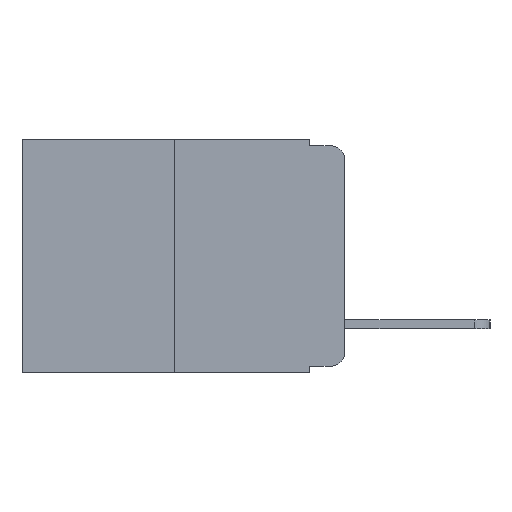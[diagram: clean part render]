
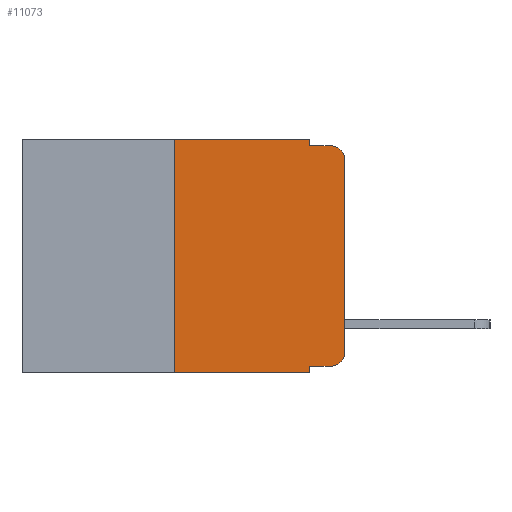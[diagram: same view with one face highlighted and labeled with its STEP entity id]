
A CAD part, left-side view. The second image highlights one B-rep face of the part: STEP entity #11073.
In plain terms, the highlighted planar face has unit normal (-1, 0, 0).
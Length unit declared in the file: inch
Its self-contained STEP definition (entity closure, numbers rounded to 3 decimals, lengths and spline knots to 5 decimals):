
#150 = CARTESIAN_POINT ( 'NONE',  ( 0., 0.051, -0.333 ) ) ;
#694 = CARTESIAN_POINT ( 'NONE',  ( 0., 0.051, -0.343 ) ) ;
#814 = DIRECTION ( 'NONE',  ( 0., -1., 0. ) ) ;
#2095 = DIRECTION ( 'NONE',  ( 0., -1., 0. ) ) ;
#2851 = LINE ( 'NONE', #6219, #6591 ) ;
#3187 = VERTEX_POINT ( 'NONE', #4512 ) ;
#4358 = EDGE_CURVE ( 'NONE', #10413, #14673, #15029, .T. ) ;
#4512 = CARTESIAN_POINT ( 'NONE',  ( 0., 0.051, -0.333 ) ) ;
#5055 = DIRECTION ( 'NONE',  ( 0., -1., 0. ) ) ;
#5499 = VERTEX_POINT ( 'NONE', #18610 ) ;
#5692 = LINE ( 'NONE', #6854, #15214 ) ;
#6219 = CARTESIAN_POINT ( 'NONE',  ( 0., 0.473, 0. ) ) ;
#6591 = VECTOR ( 'NONE', #15666, 39.37008 ) ;
#6714 = CARTESIAN_POINT ( 'NONE',  ( 0., 0., -0.03 ) ) ;
#6854 = CARTESIAN_POINT ( 'NONE',  ( 0., 0.473, -0.343 ) ) ;
#7719 = CARTESIAN_POINT ( 'NONE',  ( 0., 0.02, -0.03 ) ) ;
#7760 = ORIENTED_EDGE ( 'NONE', *, *, #13762, .T. ) ;
#7938 = ORIENTED_EDGE ( 'NONE', *, *, #14966, .T. ) ;
#8067 = ORIENTED_EDGE ( 'NONE', *, *, #16184, .F. ) ;
#8195 = ORIENTED_EDGE ( 'NONE', *, *, #19721, .F. ) ;
#8263 = DIRECTION ( 'NONE',  ( 0., 0., -1. ) ) ;
#8351 = ORIENTED_EDGE ( 'NONE', *, *, #21509, .F. ) ;
#8420 = VECTOR ( 'NONE', #19417, 39.37008 ) ;
#8517 = CARTESIAN_POINT ( 'NONE',  ( 0., 0.25, 0. ) ) ;
#8689 = LINE ( 'NONE', #17704, #18044 ) ;
#8781 = ORIENTED_EDGE ( 'NONE', *, *, #4358, .F. ) ;
#8802 = ORIENTED_EDGE ( 'NONE', *, *, #21720, .T. ) ;
#8980 = ORIENTED_EDGE ( 'NONE', *, *, #10697, .F. ) ;
#9403 = ORIENTED_EDGE ( 'NONE', *, *, #10216, .T. ) ;
#9608 = ORIENTED_EDGE ( 'NONE', *, *, #9860, .T. ) ;
#9687 = DIRECTION ( 'NONE',  ( 0., 0., -1. ) ) ;
#9860 = EDGE_CURVE ( 'NONE', #12364, #5499, #10754, .T. ) ;
#9892 = CARTESIAN_POINT ( 'NONE',  ( 0., 0.473, 0. ) ) ;
#10216 = EDGE_CURVE ( 'NONE', #3187, #12364, #19319, .T. ) ;
#10413 = VERTEX_POINT ( 'NONE', #12498 ) ;
#10498 = DIRECTION ( 'NONE',  ( 0., 0., 1. ) ) ;
#10518 = EDGE_LOOP ( 'NONE', ( #7760, #7938, #8067, #8195, #8351, #8781, #8802, #8980, #9403, #9608 ) ) ;
#10697 = EDGE_CURVE ( 'NONE', #3187, #17299, #8689, .T. ) ;
#10754 = CIRCLE ( 'NONE', #13835, 0.02 ) ;
#10838 = CARTESIAN_POINT ( 'NONE',  ( 0., 0., 0. ) ) ;
#11073 = ADVANCED_FACE ( 'NONE', ( #19143 ), #20799, .F. ) ;
#11383 = DIRECTION ( 'NONE',  ( -1., 0., 0. ) ) ;
#11640 = AXIS2_PLACEMENT_3D ( 'NONE', #9892, #22501, #11846 ) ;
#11846 = DIRECTION ( 'NONE',  ( 0., 0., -1. ) ) ;
#12173 = DIRECTION ( 'NONE',  ( 0., 0., -1. ) ) ;
#12201 = CARTESIAN_POINT ( 'NONE',  ( 0., 0.051, -0.01 ) ) ;
#12364 = VERTEX_POINT ( 'NONE', #14083 ) ;
#12498 = CARTESIAN_POINT ( 'NONE',  ( 0., 0.25, -0.343 ) ) ;
#12636 = CARTESIAN_POINT ( 'NONE',  ( 0., 0.25, 0. ) ) ;
#13213 = VERTEX_POINT ( 'NONE', #14262 ) ;
#13762 = EDGE_CURVE ( 'NONE', #5499, #20594, #17662, .T. ) ;
#13835 = AXIS2_PLACEMENT_3D ( 'NONE', #22118, #11383, #12173 ) ;
#14083 = CARTESIAN_POINT ( 'NONE',  ( 0., 0.02, -0.333 ) ) ;
#14163 = LINE ( 'NONE', #21128, #8420 ) ;
#14262 = CARTESIAN_POINT ( 'NONE',  ( 0., 0.051, 0. ) ) ;
#14574 = VECTOR ( 'NONE', #2095, 39.37008 ) ;
#14673 = VERTEX_POINT ( 'NONE', #12636 ) ;
#14966 = EDGE_CURVE ( 'NONE', #20594, #16890, #17603, .T. ) ;
#15012 = VERTEX_POINT ( 'NONE', #17270 ) ;
#15029 = LINE ( 'NONE', #8517, #23692 ) ;
#15214 = VECTOR ( 'NONE', #5055, 39.37008 ) ;
#15666 = DIRECTION ( 'NONE',  ( 0., -1., 0. ) ) ;
#15860 = VECTOR ( 'NONE', #814, 39.37008 ) ;
#16184 = EDGE_CURVE ( 'NONE', #15012, #16890, #19993, .T. ) ;
#16391 = DIRECTION ( 'NONE',  ( 0., 0., 1. ) ) ;
#16580 = AXIS2_PLACEMENT_3D ( 'NONE', #7719, #20627, #9687 ) ;
#16890 = VERTEX_POINT ( 'NONE', #18285 ) ;
#17270 = CARTESIAN_POINT ( 'NONE',  ( 0., 0.051, -0.01 ) ) ;
#17299 = VERTEX_POINT ( 'NONE', #694 ) ;
#17603 = CIRCLE ( 'NONE', #16580, 0.02 ) ;
#17662 = LINE ( 'NONE', #10838, #22264 ) ;
#17704 = CARTESIAN_POINT ( 'NONE',  ( 0., 0.051, 0. ) ) ;
#18044 = VECTOR ( 'NONE', #8263, 39.37008 ) ;
#18285 = CARTESIAN_POINT ( 'NONE',  ( 0., 0.02, -0.01 ) ) ;
#18610 = CARTESIAN_POINT ( 'NONE',  ( 0., 0., -0.313 ) ) ;
#19143 = FACE_OUTER_BOUND ( 'NONE', #10518, .T. ) ;
#19319 = LINE ( 'NONE', #150, #14574 ) ;
#19417 = DIRECTION ( 'NONE',  ( 0., 0., -1. ) ) ;
#19721 = EDGE_CURVE ( 'NONE', #13213, #15012, #14163, .T. ) ;
#19993 = LINE ( 'NONE', #12201, #15860 ) ;
#20594 = VERTEX_POINT ( 'NONE', #6714 ) ;
#20627 = DIRECTION ( 'NONE',  ( -1., 0., 0. ) ) ;
#20799 = PLANE ( 'NONE',  #11640 ) ;
#21128 = CARTESIAN_POINT ( 'NONE',  ( 0., 0.051, 0. ) ) ;
#21509 = EDGE_CURVE ( 'NONE', #14673, #13213, #2851, .T. ) ;
#21720 = EDGE_CURVE ( 'NONE', #10413, #17299, #5692, .T. ) ;
#22118 = CARTESIAN_POINT ( 'NONE',  ( 0., 0.02, -0.313 ) ) ;
#22264 = VECTOR ( 'NONE', #16391, 39.37008 ) ;
#22501 = DIRECTION ( 'NONE',  ( 1., 0., 0. ) ) ;
#23692 = VECTOR ( 'NONE', #10498, 39.37008 ) ;
